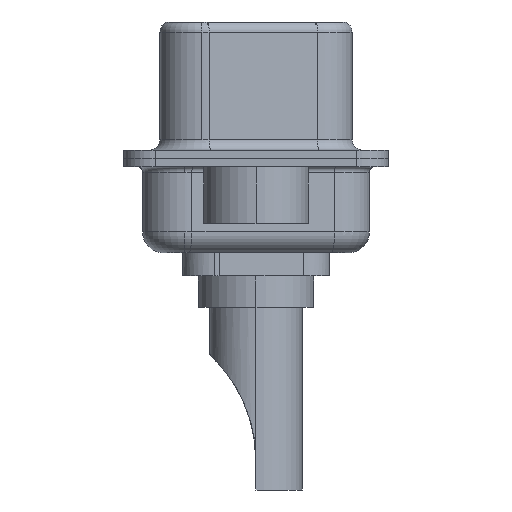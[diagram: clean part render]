
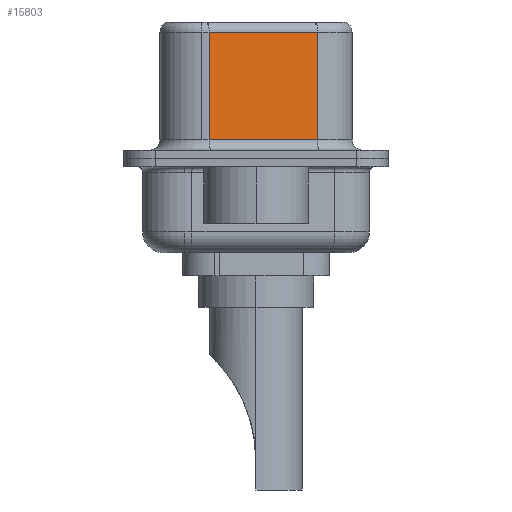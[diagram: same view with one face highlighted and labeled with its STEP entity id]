
A CAD part, left-side view. The second image highlights one B-rep face of the part: STEP entity #15803.
In plain terms, the highlighted planar face has unit normal (-0.985, -0.174, 0).
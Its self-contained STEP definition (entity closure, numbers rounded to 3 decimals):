
#198 = VECTOR ( 'NONE', #3655, 1000. ) ;
#1690 = ORIENTED_EDGE ( 'NONE', *, *, #17555, .T. ) ;
#2259 = ORIENTED_EDGE ( 'NONE', *, *, #18071, .F. ) ;
#2380 = ORIENTED_EDGE ( 'NONE', *, *, #11989, .T. ) ;
#3272 = VECTOR ( 'NONE', #10075, 1000. ) ;
#3655 = DIRECTION ( 'NONE',  ( 0., 0., -1. ) ) ;
#3895 = CARTESIAN_POINT ( 'NONE',  ( 4.58, -2.927, 0.9 ) ) ;
#4614 = VERTEX_POINT ( 'NONE', #9629 ) ;
#4624 = FACE_OUTER_BOUND ( 'NONE', #15717, .T. ) ;
#5780 = CARTESIAN_POINT ( 'NONE',  ( 3.67, 2.233, 6.52 ) ) ;
#8453 = EDGE_CURVE ( 'NONE', #14051, #20446, #14713, .T. ) ;
#8494 = CARTESIAN_POINT ( 'NONE',  ( 3.67, 2.233, 0.9 ) ) ;
#8691 = VECTOR ( 'NONE', #21756, 1000. ) ;
#8858 = DIRECTION ( 'NONE',  ( 0.985, 0.174, 0. ) ) ;
#9445 = VECTOR ( 'NONE', #23646, 1000. ) ;
#9629 = CARTESIAN_POINT ( 'NONE',  ( 4.58, -2.927, 0.9 ) ) ;
#9880 = CARTESIAN_POINT ( 'NONE',  ( 4.58, -2.927, 6.02 ) ) ;
#10075 = DIRECTION ( 'NONE',  ( -0.174, 0.985, 0. ) ) ;
#11621 = CARTESIAN_POINT ( 'NONE',  ( 4.58, -2.927, 6.52 ) ) ;
#11989 = EDGE_CURVE ( 'NONE', #20446, #4614, #18527, .T. ) ;
#12372 = ORIENTED_EDGE ( 'NONE', *, *, #8453, .T. ) ;
#14051 = VERTEX_POINT ( 'NONE', #19549 ) ;
#14713 = LINE ( 'NONE', #5780, #9445 ) ;
#15471 = LINE ( 'NONE', #11621, #198 ) ;
#15717 = EDGE_LOOP ( 'NONE', ( #2259, #1690, #12372, #2380 ) ) ;
#15803 = ADVANCED_FACE ( 'NONE', ( #4624 ), #22625, .F. ) ;
#17555 = EDGE_CURVE ( 'NONE', #18314, #14051, #19100, .T. ) ;
#17988 = CARTESIAN_POINT ( 'NONE',  ( 4.58, -2.927, 6.02 ) ) ;
#18071 = EDGE_CURVE ( 'NONE', #18314, #4614, #15471, .T. ) ;
#18314 = VERTEX_POINT ( 'NONE', #9880 ) ;
#18527 = LINE ( 'NONE', #3895, #8691 ) ;
#19100 = LINE ( 'NONE', #17988, #3272 ) ;
#19549 = CARTESIAN_POINT ( 'NONE',  ( 3.67, 2.233, 6.02 ) ) ;
#20446 = VERTEX_POINT ( 'NONE', #8494 ) ;
#20655 = CARTESIAN_POINT ( 'NONE',  ( 4.58, -2.927, 6.52 ) ) ;
#21756 = DIRECTION ( 'NONE',  ( 0.174, -0.985, 0. ) ) ;
#22625 = PLANE ( 'NONE',  #24016 ) ;
#22716 = DIRECTION ( 'NONE',  ( -0.174, 0.985, 0. ) ) ;
#23646 = DIRECTION ( 'NONE',  ( 0., 0., -1. ) ) ;
#24016 = AXIS2_PLACEMENT_3D ( 'NONE', #20655, #8858, #22716 ) ;
